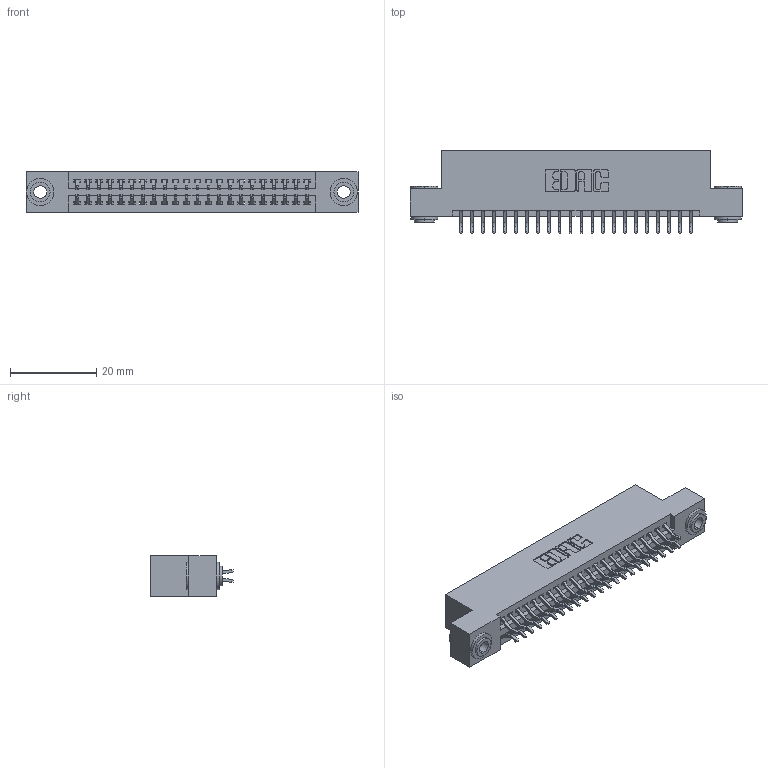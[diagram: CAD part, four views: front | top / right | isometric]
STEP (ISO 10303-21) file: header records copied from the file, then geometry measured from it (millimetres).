
FILE_DESCRIPTION (( 'STEP AP203' ), '1' );
FILE_NAME ('395-044-556-203.STEP', '2018-11-15T21:59:01', ( '' ), ( '' ), 'SwSTEP 2.0', 'SolidWorks 2016', '' );
FILE_SCHEMA (( 'CONFIG_CONTROL_DESIGN' ));
Length unit declared in the file: inch
Products named in the file (4): 345 Part_Flush Mounting Lugs - 0.156 Dia-TH; 395-044-556-203; 345-292-001_556 Tail; 345-250-002_345-250-002-102
Assembly tree (47 placements, depth 2):
  395-044-556-203
    345 Part_Flush Mounting Lugs - 0.156 Dia-TH
    345-292-001_556 Tail  x44
    345-250-002_345-250-002-102  x2
Bounding box: 77.09 x 19.24 x 9.4 mm (x, y, z)
Volume: 7320.5 mm3; surface area: 10600 mm2
Topology: 47 solids, 47 shells, 2628 faces, 7765 edges, 5114 vertices
Faces by surface type: plane 1718, cylinder 902, cone 8
Entity records: 20824 total; most frequent: CARTESIAN_POINT 3499, ORIENTED_EDGE 3414, DIRECTION 3129, EDGE_CURVE 1707, LINE 1455, VECTOR 1455, VERTEX_POINT 1134, AXIS2_PLACEMENT_3D 837
